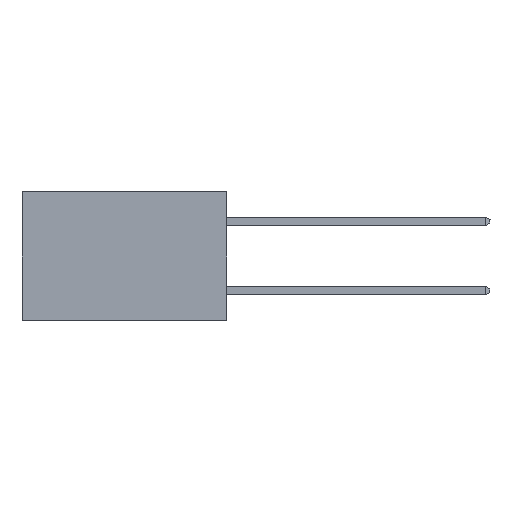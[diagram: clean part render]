
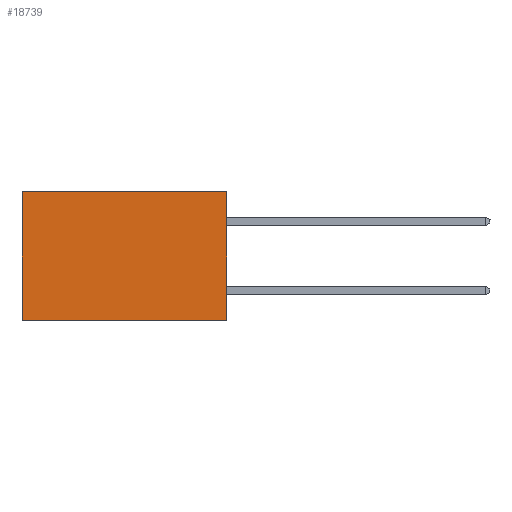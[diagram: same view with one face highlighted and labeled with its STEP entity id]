
A CAD part, left-side view. The second image highlights one B-rep face of the part: STEP entity #18739.
In plain terms, the highlighted planar face has unit normal (-1, 0, 0).
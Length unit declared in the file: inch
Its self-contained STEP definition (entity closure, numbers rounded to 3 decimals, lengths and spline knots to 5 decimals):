
#331 = AXIS2_PLACEMENT_3D ( 'NONE', #854, #3186, #19124 ) ;
#854 = CARTESIAN_POINT ( 'NONE',  ( 0.277, 0., -0.37 ) ) ;
#1559 = EDGE_CURVE ( 'NONE', #6400, #25505, #4031, .T. ) ;
#1924 = VECTOR ( 'NONE', #4088, 39.37008 ) ;
#3000 = VERTEX_POINT ( 'NONE', #19518 ) ;
#3186 = DIRECTION ( 'NONE',  ( 1., 0., 0. ) ) ;
#4031 = LINE ( 'NONE', #16827, #15406 ) ;
#4088 = DIRECTION ( 'NONE',  ( 0., 1., 0. ) ) ;
#5135 = DIRECTION ( 'NONE',  ( 0., 0., -1. ) ) ;
#5619 = EDGE_CURVE ( 'NONE', #17761, #3000, #16138, .T. ) ;
#6400 = VERTEX_POINT ( 'NONE', #14238 ) ;
#9920 = LINE ( 'NONE', #15917, #21250 ) ;
#13575 = ORIENTED_EDGE ( 'NONE', *, *, #1559, .T. ) ;
#14238 = CARTESIAN_POINT ( 'NONE',  ( 0.277, 0.59, 0. ) ) ;
#15406 = VECTOR ( 'NONE', #5135, 39.37008 ) ;
#15607 = EDGE_CURVE ( 'NONE', #17761, #6400, #9920, .T. ) ;
#15917 = CARTESIAN_POINT ( 'NONE',  ( 0.277, 0., 0. ) ) ;
#16138 = LINE ( 'NONE', #28448, #21452 ) ;
#16827 = CARTESIAN_POINT ( 'NONE',  ( 0.277, 0.59, -0.37 ) ) ;
#16841 = PLANE ( 'NONE',  #331 ) ;
#16904 = ORIENTED_EDGE ( 'NONE', *, *, #15607, .T. ) ;
#17473 = EDGE_CURVE ( 'NONE', #3000, #25505, #25354, .T. ) ;
#17761 = VERTEX_POINT ( 'NONE', #27295 ) ;
#18201 = DIRECTION ( 'NONE',  ( 0., 1., 0. ) ) ;
#18739 = ADVANCED_FACE ( 'NONE', ( #23567 ), #16841, .F. ) ;
#19124 = DIRECTION ( 'NONE',  ( 0., 0., -1. ) ) ;
#19518 = CARTESIAN_POINT ( 'NONE',  ( 0.277, 0., -0.37 ) ) ;
#20929 = ORIENTED_EDGE ( 'NONE', *, *, #17473, .F. ) ;
#21250 = VECTOR ( 'NONE', #18201, 39.37008 ) ;
#21452 = VECTOR ( 'NONE', #29152, 39.37008 ) ;
#21570 = ORIENTED_EDGE ( 'NONE', *, *, #5619, .F. ) ;
#21835 = EDGE_LOOP ( 'NONE', ( #13575, #20929, #21570, #16904 ) ) ;
#23567 = FACE_OUTER_BOUND ( 'NONE', #21835, .T. ) ;
#25354 = LINE ( 'NONE', #26551, #1924 ) ;
#25505 = VERTEX_POINT ( 'NONE', #27731 ) ;
#26551 = CARTESIAN_POINT ( 'NONE',  ( 0.277, 0., -0.37 ) ) ;
#27295 = CARTESIAN_POINT ( 'NONE',  ( 0.277, 0., 0. ) ) ;
#27731 = CARTESIAN_POINT ( 'NONE',  ( 0.277, 0.59, -0.37 ) ) ;
#28448 = CARTESIAN_POINT ( 'NONE',  ( 0.277, 0., -0.37 ) ) ;
#29152 = DIRECTION ( 'NONE',  ( 0., 0., -1. ) ) ;
